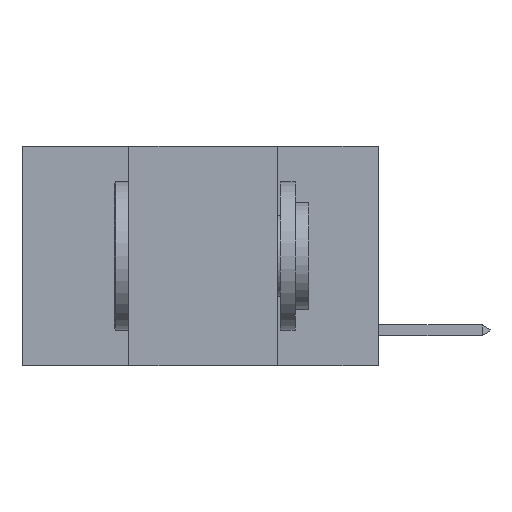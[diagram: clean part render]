
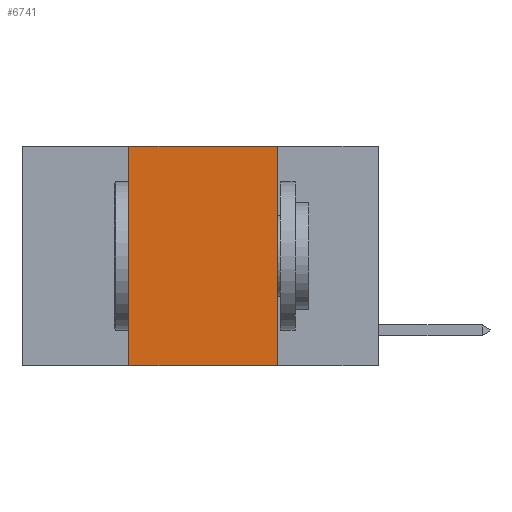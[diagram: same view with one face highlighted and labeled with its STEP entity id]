
A CAD part, left-side view. The second image highlights one B-rep face of the part: STEP entity #6741.
In plain terms, the highlighted planar face has unit normal (-1, 0, 0).
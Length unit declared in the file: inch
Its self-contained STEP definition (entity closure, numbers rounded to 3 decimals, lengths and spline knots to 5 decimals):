
#90 = EDGE_CURVE ( 'NONE', #27061, #27267, #20496, .T. ) ;
#519 = ORIENTED_EDGE ( 'NONE', *, *, #5481, .F. ) ;
#903 = DIRECTION ( 'NONE',  ( 0., 0., 1. ) ) ;
#1178 = DIRECTION ( 'NONE',  ( 0., 0., -1. ) ) ;
#1612 = CARTESIAN_POINT ( 'NONE',  ( 0., 0.17, 0. ) ) ;
#2056 = CARTESIAN_POINT ( 'NONE',  ( 0., 0.17, 0. ) ) ;
#4445 = CARTESIAN_POINT ( 'NONE',  ( 0., 0.42, -0.37 ) ) ;
#5481 = EDGE_CURVE ( 'NONE', #19332, #27061, #18201, .T. ) ;
#5987 = LINE ( 'NONE', #12116, #28909 ) ;
#6741 = ADVANCED_FACE ( 'NONE', ( #6986 ), #10075, .F. ) ;
#6986 = FACE_OUTER_BOUND ( 'NONE', #27538, .T. ) ;
#7886 = EDGE_CURVE ( 'NONE', #15897, #27267, #10403, .T. ) ;
#7933 = VECTOR ( 'NONE', #1178, 39.37008 ) ;
#8617 = ORIENTED_EDGE ( 'NONE', *, *, #17395, .F. ) ;
#8643 = ORIENTED_EDGE ( 'NONE', *, *, #7886, .T. ) ;
#10075 = PLANE ( 'NONE',  #11638 ) ;
#10403 = LINE ( 'NONE', #16632, #21536 ) ;
#11303 = CARTESIAN_POINT ( 'NONE',  ( 0., 0.17, -0.37 ) ) ;
#11638 = AXIS2_PLACEMENT_3D ( 'NONE', #12318, #27803, #14556 ) ;
#11793 = ORIENTED_EDGE ( 'NONE', *, *, #90, .F. ) ;
#12116 = CARTESIAN_POINT ( 'NONE',  ( 0., 0.42, 0. ) ) ;
#12264 = DIRECTION ( 'NONE',  ( 0., -1., 0. ) ) ;
#12318 = CARTESIAN_POINT ( 'NONE',  ( 0., 0.6, 0. ) ) ;
#13916 = DIRECTION ( 'NONE',  ( 0., -1., 0. ) ) ;
#14556 = DIRECTION ( 'NONE',  ( 0., 0., -1. ) ) ;
#15897 = VERTEX_POINT ( 'NONE', #4445 ) ;
#16325 = CARTESIAN_POINT ( 'NONE',  ( 0., 0.42, 0. ) ) ;
#16632 = CARTESIAN_POINT ( 'NONE',  ( 0., 0.6, -0.37 ) ) ;
#17395 = EDGE_CURVE ( 'NONE', #15897, #19332, #5987, .T. ) ;
#18201 = LINE ( 'NONE', #20616, #21345 ) ;
#19332 = VERTEX_POINT ( 'NONE', #16325 ) ;
#20496 = LINE ( 'NONE', #2056, #7933 ) ;
#20616 = CARTESIAN_POINT ( 'NONE',  ( 0., 0.6, 0. ) ) ;
#21345 = VECTOR ( 'NONE', #13916, 39.37008 ) ;
#21536 = VECTOR ( 'NONE', #12264, 39.37008 ) ;
#27061 = VERTEX_POINT ( 'NONE', #1612 ) ;
#27267 = VERTEX_POINT ( 'NONE', #11303 ) ;
#27538 = EDGE_LOOP ( 'NONE', ( #11793, #519, #8617, #8643 ) ) ;
#27803 = DIRECTION ( 'NONE',  ( 1., 0., 0. ) ) ;
#28909 = VECTOR ( 'NONE', #903, 39.37008 ) ;
